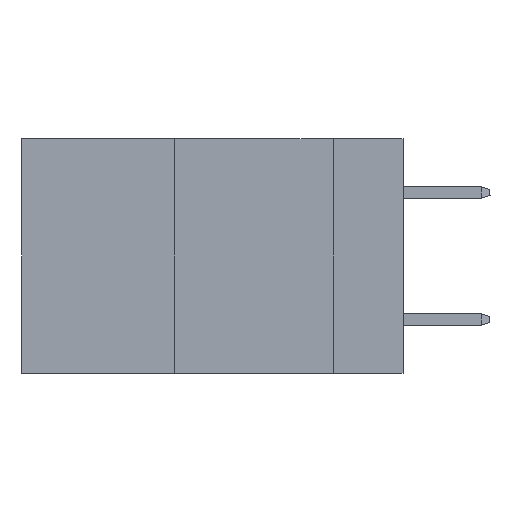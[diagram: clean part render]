
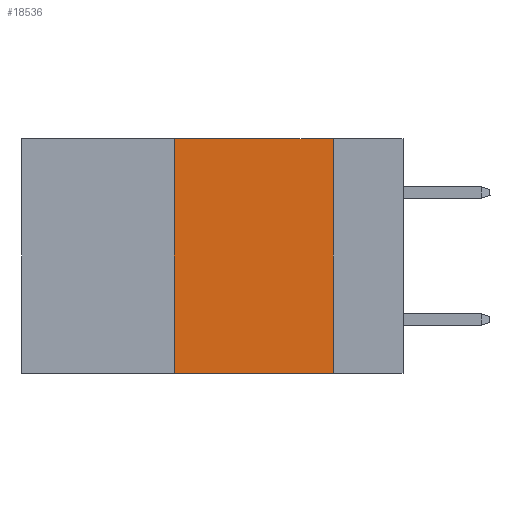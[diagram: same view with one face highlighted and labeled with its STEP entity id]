
A CAD part, left-side view. The second image highlights one B-rep face of the part: STEP entity #18536.
In plain terms, the highlighted planar face has unit normal (-1, 0, 0).
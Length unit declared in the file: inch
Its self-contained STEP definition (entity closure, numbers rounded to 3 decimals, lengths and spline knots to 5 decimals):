
#780 = FACE_OUTER_BOUND ( 'NONE', #11472, .T. ) ;
#1530 = DIRECTION ( 'NONE',  ( 0., 0., -1. ) ) ;
#1541 = VERTEX_POINT ( 'NONE', #17342 ) ;
#1665 = CARTESIAN_POINT ( 'NONE',  ( 0., 0.11, -0.37 ) ) ;
#3184 = EDGE_CURVE ( 'NONE', #10530, #1541, #6703, .T. ) ;
#3568 = EDGE_CURVE ( 'NONE', #21015, #10530, #19993, .T. ) ;
#3876 = EDGE_CURVE ( 'NONE', #21015, #15182, #7231, .T. ) ;
#4205 = DIRECTION ( 'NONE',  ( 1., 0., 0. ) ) ;
#4222 = CARTESIAN_POINT ( 'NONE',  ( 0., 0.36, 0. ) ) ;
#4296 = VECTOR ( 'NONE', #15115, 39.37008 ) ;
#5393 = CARTESIAN_POINT ( 'NONE',  ( 0., 0.36, -0.37 ) ) ;
#6703 = LINE ( 'NONE', #13695, #4296 ) ;
#6925 = VECTOR ( 'NONE', #7810, 39.37008 ) ;
#7231 = LINE ( 'NONE', #7356, #8748 ) ;
#7356 = CARTESIAN_POINT ( 'NONE',  ( 0., 0.6, -0.37 ) ) ;
#7810 = DIRECTION ( 'NONE',  ( 0., 0., 1. ) ) ;
#8748 = VECTOR ( 'NONE', #8952, 39.37008 ) ;
#8952 = DIRECTION ( 'NONE',  ( 0., -1., 0. ) ) ;
#9981 = DIRECTION ( 'NONE',  ( 0., 0., -1. ) ) ;
#10307 = LINE ( 'NONE', #17316, #19430 ) ;
#10530 = VERTEX_POINT ( 'NONE', #14011 ) ;
#11063 = PLANE ( 'NONE',  #17185 ) ;
#11472 = EDGE_LOOP ( 'NONE', ( #13211, #14032, #18579, #17597 ) ) ;
#13211 = ORIENTED_EDGE ( 'NONE', *, *, #20725, .F. ) ;
#13695 = CARTESIAN_POINT ( 'NONE',  ( 0., 0.6, 0. ) ) ;
#14011 = CARTESIAN_POINT ( 'NONE',  ( 0., 0.36, 0. ) ) ;
#14032 = ORIENTED_EDGE ( 'NONE', *, *, #3184, .F. ) ;
#15115 = DIRECTION ( 'NONE',  ( 0., -1., 0. ) ) ;
#15182 = VERTEX_POINT ( 'NONE', #1665 ) ;
#17185 = AXIS2_PLACEMENT_3D ( 'NONE', #18062, #4205, #9981 ) ;
#17316 = CARTESIAN_POINT ( 'NONE',  ( 0., 0.11, 0. ) ) ;
#17342 = CARTESIAN_POINT ( 'NONE',  ( 0., 0.11, 0. ) ) ;
#17597 = ORIENTED_EDGE ( 'NONE', *, *, #3876, .T. ) ;
#18062 = CARTESIAN_POINT ( 'NONE',  ( 0., 0.6, 0. ) ) ;
#18536 = ADVANCED_FACE ( 'NONE', ( #780 ), #11063, .F. ) ;
#18579 = ORIENTED_EDGE ( 'NONE', *, *, #3568, .F. ) ;
#19430 = VECTOR ( 'NONE', #1530, 39.37008 ) ;
#19993 = LINE ( 'NONE', #4222, #6925 ) ;
#20725 = EDGE_CURVE ( 'NONE', #1541, #15182, #10307, .T. ) ;
#21015 = VERTEX_POINT ( 'NONE', #5393 ) ;
